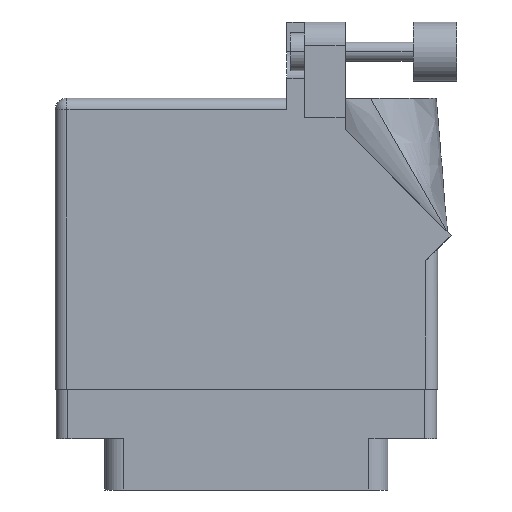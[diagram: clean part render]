
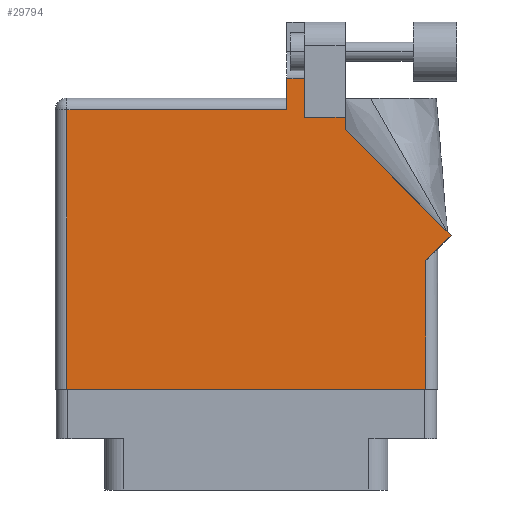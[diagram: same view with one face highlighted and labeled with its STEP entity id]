
A CAD part, front view. The second image highlights one B-rep face of the part: STEP entity #29794.
In plain terms, the highlighted face is planar.
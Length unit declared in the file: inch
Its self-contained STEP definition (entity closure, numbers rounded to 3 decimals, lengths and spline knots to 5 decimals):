
#152 = EDGE_CURVE ( 'NONE', #362, #11702, #20360, .T. ) ;
#357 = CARTESIAN_POINT ( 'NONE',  ( 0.062, 0., 0. ) ) ;
#362 = VERTEX_POINT ( 'NONE', #15622 ) ;
#752 = DIRECTION ( 'NONE',  ( 1., 0., 0. ) ) ;
#2051 = LINE ( 'NONE', #15888, #17263 ) ;
#2172 = CARTESIAN_POINT ( 'NONE',  ( 1.217, 1.468, 0. ) ) ;
#2376 = EDGE_CURVE ( 'NONE', #37820, #2994, #3499, .T. ) ;
#2507 = EDGE_CURVE ( 'NONE', #35520, #37820, #35789, .T. ) ;
#2994 = VERTEX_POINT ( 'NONE', #2172 ) ;
#3499 = LINE ( 'NONE', #15611, #38619 ) ;
#3548 = DIRECTION ( 'NONE',  ( 0., 1., 0. ) ) ;
#3826 = CARTESIAN_POINT ( 'NONE',  ( 1.311, 1.6315, 0. ) ) ;
#4114 = CARTESIAN_POINT ( 'NONE',  ( 1.64177, 1.6315, 0. ) ) ;
#4898 = EDGE_CURVE ( 'NONE', #21569, #19215, #5676, .T. ) ;
#5293 = LINE ( 'NONE', #7011, #35674 ) ;
#5676 = LINE ( 'NONE', #32003, #9908 ) ;
#7011 = CARTESIAN_POINT ( 'NONE',  ( 0.062, 0., 0. ) ) ;
#7123 = ORIENTED_EDGE ( 'NONE', *, *, #4898, .T. ) ;
#7306 = ORIENTED_EDGE ( 'NONE', *, *, #19283, .T. ) ;
#7715 = DIRECTION ( 'NONE',  ( 0., 1., 0. ) ) ;
#7840 = VECTOR ( 'NONE', #25648, 39.37008 ) ;
#8039 = ORIENTED_EDGE ( 'NONE', *, *, #9538, .T. ) ;
#8242 = VERTEX_POINT ( 'NONE', #27254 ) ;
#8459 = PLANE ( 'NONE',  #13024 ) ;
#8500 = ORIENTED_EDGE ( 'NONE', *, *, #22858, .T. ) ;
#8825 = DIRECTION ( 'NONE',  ( 0., 1., 0. ) ) ;
#9088 = VECTOR ( 'NONE', #23328, 39.37008 ) ;
#9144 = EDGE_CURVE ( 'NONE', #19215, #362, #32068, .T. ) ;
#9500 = CARTESIAN_POINT ( 'NONE',  ( 1.948, 0., 0. ) ) ;
#9538 = EDGE_CURVE ( 'NONE', #8242, #35520, #25909, .T. ) ;
#9908 = VECTOR ( 'NONE', #7715, 39.37008 ) ;
#9935 = ORIENTED_EDGE ( 'NONE', *, *, #152, .T. ) ;
#10028 = DIRECTION ( 'NONE',  ( 0., -1., 0. ) ) ;
#10596 = VECTOR ( 'NONE', #26151, 39.37008 ) ;
#11702 = VERTEX_POINT ( 'NONE', #13212 ) ;
#12331 = CARTESIAN_POINT ( 'NONE',  ( 0.062, 1.468, 0. ) ) ;
#13024 = AXIS2_PLACEMENT_3D ( 'NONE', #14851, #29853, #26949 ) ;
#13212 = CARTESIAN_POINT ( 'NONE',  ( 1.524, 1.36442, 0. ) ) ;
#14851 = CARTESIAN_POINT ( 'NONE',  ( 0., 1.53, 0. ) ) ;
#14880 = EDGE_CURVE ( 'NONE', #11702, #38713, #23513, .T. ) ;
#15485 = CARTESIAN_POINT ( 'NONE',  ( 1.311, 1.43, 0. ) ) ;
#15611 = CARTESIAN_POINT ( 'NONE',  ( 1.217, 1.53, 0. ) ) ;
#15622 = CARTESIAN_POINT ( 'NONE',  ( 2.08071, 0.80771, 0. ) ) ;
#15888 = CARTESIAN_POINT ( 'NONE',  ( 0., 0., 0. ) ) ;
#15903 = ORIENTED_EDGE ( 'NONE', *, *, #16644, .T. ) ;
#16332 = CARTESIAN_POINT ( 'NONE',  ( 2.01, 0.737, 0. ) ) ;
#16644 = EDGE_CURVE ( 'NONE', #25275, #35788, #5293, .T. ) ;
#17263 = VECTOR ( 'NONE', #752, 39.37008 ) ;
#18174 = EDGE_CURVE ( 'NONE', #2994, #25275, #18449, .T. ) ;
#18188 = CARTESIAN_POINT ( 'NONE',  ( 1.524, 1.36442, 0. ) ) ;
#18449 = LINE ( 'NONE', #23018, #23252 ) ;
#19215 = VERTEX_POINT ( 'NONE', #19617 ) ;
#19283 = EDGE_CURVE ( 'NONE', #38713, #8242, #19624, .T. ) ;
#19617 = CARTESIAN_POINT ( 'NONE',  ( 1.948, 0.675, 0. ) ) ;
#19624 = LINE ( 'NONE', #38890, #9088 ) ;
#19845 = ORIENTED_EDGE ( 'NONE', *, *, #2507, .T. ) ;
#20291 = ORIENTED_EDGE ( 'NONE', *, *, #14880, .T. ) ;
#20360 = LINE ( 'NONE', #31871, #29337 ) ;
#20731 = ORIENTED_EDGE ( 'NONE', *, *, #2376, .T. ) ;
#21149 = VECTOR ( 'NONE', #8825, 39.37008 ) ;
#21569 = VERTEX_POINT ( 'NONE', #9500 ) ;
#21600 = DIRECTION ( 'NONE',  ( 0., -1., 0. ) ) ;
#22858 = EDGE_CURVE ( 'NONE', #35788, #21569, #2051, .T. ) ;
#23018 = CARTESIAN_POINT ( 'NONE',  ( 0., 1.468, 0. ) ) ;
#23252 = VECTOR ( 'NONE', #26421, 39.37008 ) ;
#23328 = DIRECTION ( 'NONE',  ( -1., 0., 0. ) ) ;
#23513 = LINE ( 'NONE', #18188, #37677 ) ;
#24122 = ORIENTED_EDGE ( 'NONE', *, *, #18174, .T. ) ;
#25275 = VERTEX_POINT ( 'NONE', #12331 ) ;
#25648 = DIRECTION ( 'NONE',  ( 0.707, 0.707, 0. ) ) ;
#25909 = LINE ( 'NONE', #15485, #21149 ) ;
#26151 = DIRECTION ( 'NONE',  ( -1., 0., 0. ) ) ;
#26421 = DIRECTION ( 'NONE',  ( -1., 0., 0. ) ) ;
#26949 = DIRECTION ( 'NONE',  ( -1., 0., 0. ) ) ;
#27254 = CARTESIAN_POINT ( 'NONE',  ( 1.311, 1.43, 0. ) ) ;
#29337 = VECTOR ( 'NONE', #36346, 39.37008 ) ;
#29794 = ADVANCED_FACE ( 'NONE', ( #31993 ), #8459, .F. ) ;
#29853 = DIRECTION ( 'NONE',  ( 0., 0., -1. ) ) ;
#31871 = CARTESIAN_POINT ( 'NONE',  ( 2.08071, 0.80771, 0. ) ) ;
#31993 = FACE_OUTER_BOUND ( 'NONE', #33165, .T. ) ;
#32003 = CARTESIAN_POINT ( 'NONE',  ( 1.948, 0.737, 0. ) ) ;
#32068 = LINE ( 'NONE', #16332, #7840 ) ;
#33165 = EDGE_LOOP ( 'NONE', ( #8039, #19845, #20731, #24122, #15903, #8500, #7123, #36561, #9935, #20291, #7306 ) ) ;
#35520 = VERTEX_POINT ( 'NONE', #3826 ) ;
#35674 = VECTOR ( 'NONE', #10028, 39.37008 ) ;
#35788 = VERTEX_POINT ( 'NONE', #357 ) ;
#35789 = LINE ( 'NONE', #4114, #10596 ) ;
#36346 = DIRECTION ( 'NONE',  ( -0.707, 0.707, 0. ) ) ;
#36561 = ORIENTED_EDGE ( 'NONE', *, *, #9144, .T. ) ;
#37677 = VECTOR ( 'NONE', #3548, 39.37008 ) ;
#37759 = CARTESIAN_POINT ( 'NONE',  ( 1.217, 1.6315, 0. ) ) ;
#37820 = VERTEX_POINT ( 'NONE', #37759 ) ;
#37922 = CARTESIAN_POINT ( 'NONE',  ( 1.524, 1.43, 0. ) ) ;
#38619 = VECTOR ( 'NONE', #21600, 39.37008 ) ;
#38713 = VERTEX_POINT ( 'NONE', #37922 ) ;
#38890 = CARTESIAN_POINT ( 'NONE',  ( 1.524, 1.43, 0. ) ) ;
